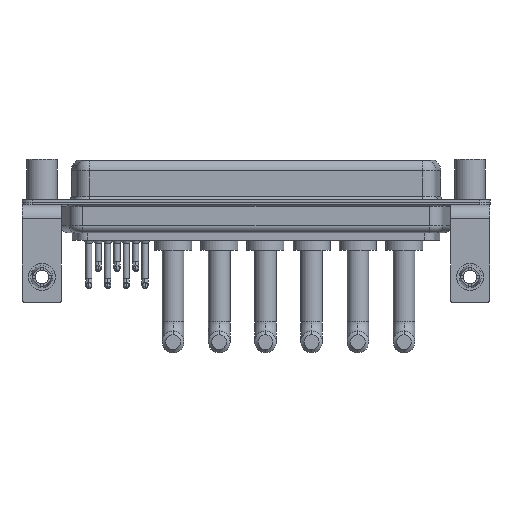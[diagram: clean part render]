
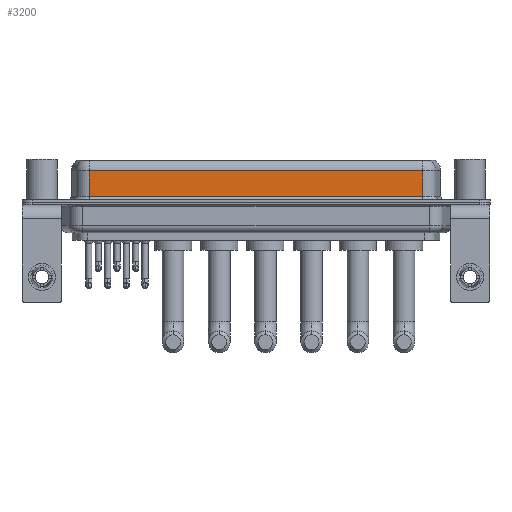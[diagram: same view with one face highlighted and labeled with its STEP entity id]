
A CAD part, front view. The second image highlights one B-rep face of the part: STEP entity #3200.
In plain terms, the highlighted planar face has unit normal (0, -1, 0).
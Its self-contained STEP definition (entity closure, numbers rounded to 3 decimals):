
#951 = EDGE_LOOP ( 'NONE', ( #4175, #3515, #20208, #13360 ) ) ;
#2057 = VERTEX_POINT ( 'NONE', #8627 ) ;
#2220 = CARTESIAN_POINT ( 'NONE',  ( 56.462, -3.95, 6.4 ) ) ;
#2240 = EDGE_CURVE ( 'NONE', #2057, #13305, #14399, .T. ) ;
#2601 = EDGE_CURVE ( 'NONE', #14221, #12980, #11921, .T. ) ;
#3200 = ADVANCED_FACE ( 'NONE', ( #7667 ), #14120, .F. ) ;
#3515 = ORIENTED_EDGE ( 'NONE', *, *, #2240, .T. ) ;
#4175 = ORIENTED_EDGE ( 'NONE', *, *, #12713, .F. ) ;
#7380 = LINE ( 'NONE', #10720, #19257 ) ;
#7564 = DIRECTION ( 'NONE',  ( 0., 0., 1. ) ) ;
#7667 = FACE_OUTER_BOUND ( 'NONE', #951, .T. ) ;
#8627 = CARTESIAN_POINT ( 'NONE',  ( 56.462, -3.95, 4.65 ) ) ;
#8705 = DIRECTION ( 'NONE',  ( 1., 0., 0. ) ) ;
#8758 = DIRECTION ( 'NONE',  ( 0., 0., -1. ) ) ;
#9287 = DIRECTION ( 'NONE',  ( -1., 0., 0. ) ) ;
#9678 = CARTESIAN_POINT ( 'NONE',  ( 7.038, -3.95, 4.65 ) ) ;
#10720 = CARTESIAN_POINT ( 'NONE',  ( 56.462, -3.95, 6.4 ) ) ;
#10939 = CARTESIAN_POINT ( 'NONE',  ( 56.462, -3.95, 4.65 ) ) ;
#11921 = LINE ( 'NONE', #18711, #13729 ) ;
#11983 = CARTESIAN_POINT ( 'NONE',  ( 7.038, -3.95, 6.4 ) ) ;
#12336 = VECTOR ( 'NONE', #8758, 1000. ) ;
#12536 = VECTOR ( 'NONE', #9287, 1000. ) ;
#12713 = EDGE_CURVE ( 'NONE', #2057, #12980, #7380, .T. ) ;
#12980 = VERTEX_POINT ( 'NONE', #20797 ) ;
#13305 = VERTEX_POINT ( 'NONE', #9678 ) ;
#13360 = ORIENTED_EDGE ( 'NONE', *, *, #2601, .T. ) ;
#13729 = VECTOR ( 'NONE', #8705, 1000. ) ;
#14120 = PLANE ( 'NONE',  #21556 ) ;
#14221 = VERTEX_POINT ( 'NONE', #18186 ) ;
#14399 = LINE ( 'NONE', #10939, #12536 ) ;
#15493 = EDGE_CURVE ( 'NONE', #13305, #14221, #16786, .T. ) ;
#16786 = LINE ( 'NONE', #11983, #12336 ) ;
#17614 = DIRECTION ( 'NONE',  ( 0., 0., -1. ) ) ;
#18186 = CARTESIAN_POINT ( 'NONE',  ( 7.038, -3.95, 0.9 ) ) ;
#18711 = CARTESIAN_POINT ( 'NONE',  ( 56.462, -3.95, 0.9 ) ) ;
#19257 = VECTOR ( 'NONE', #17614, 1000. ) ;
#20208 = ORIENTED_EDGE ( 'NONE', *, *, #15493, .T. ) ;
#20797 = CARTESIAN_POINT ( 'NONE',  ( 56.462, -3.95, 0.9 ) ) ;
#21256 = DIRECTION ( 'NONE',  ( 0., 1., 0. ) ) ;
#21556 = AXIS2_PLACEMENT_3D ( 'NONE', #2220, #21256, #7564 ) ;
